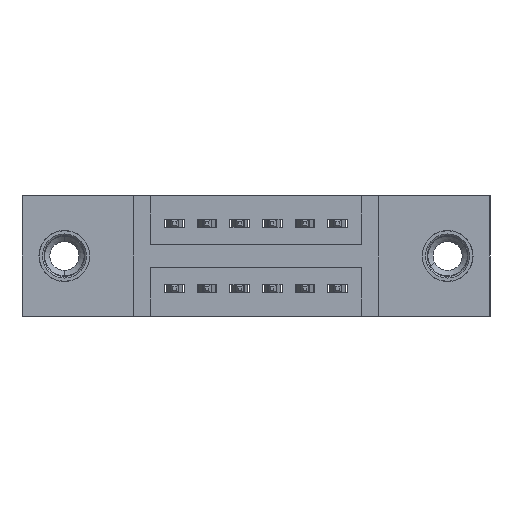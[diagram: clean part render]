
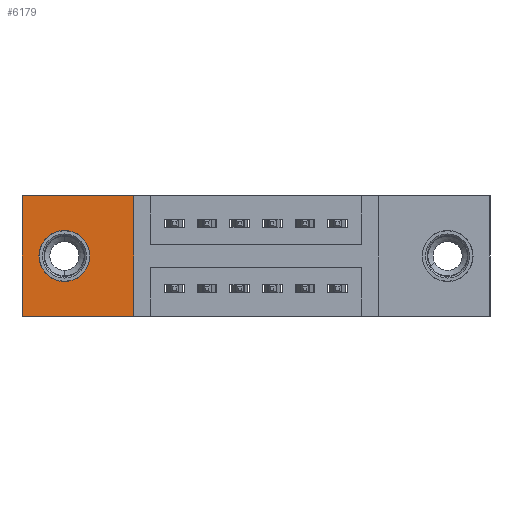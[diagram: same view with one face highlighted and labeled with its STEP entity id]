
A CAD part, front view. The second image highlights one B-rep face of the part: STEP entity #6179.
In plain terms, the highlighted planar face has unit normal (0, -1, 0).
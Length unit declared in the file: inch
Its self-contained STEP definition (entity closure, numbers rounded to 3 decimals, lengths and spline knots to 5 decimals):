
#8 = VERTEX_POINT ( 'NONE', #7902 ) ;
#120 = ORIENTED_EDGE ( 'NONE', *, *, #2230, .T. ) ;
#136 = CARTESIAN_POINT ( 'NONE',  ( 0.13, 0.17, -0.107 ) ) ;
#150 = EDGE_CURVE ( 'NONE', #256, #1971, #10466, .T. ) ;
#256 = VERTEX_POINT ( 'NONE', #9198 ) ;
#309 = EDGE_CURVE ( 'NONE', #10629, #8, #4526, .T. ) ;
#432 = CARTESIAN_POINT ( 'NONE',  ( 0.13, 0.17, -0.185 ) ) ;
#442 = DIRECTION ( 'NONE',  ( 0., 0., -1. ) ) ;
#707 = ORIENTED_EDGE ( 'NONE', *, *, #1881, .T. ) ;
#917 = EDGE_LOOP ( 'NONE', ( #5209, #6041 ) ) ;
#1339 = DIRECTION ( 'NONE',  ( 0., 0., -1. ) ) ;
#1350 = CIRCLE ( 'NONE', #8942, 0.078 ) ;
#1799 = AXIS2_PLACEMENT_3D ( 'NONE', #432, #6364, #1339 ) ;
#1854 = DIRECTION ( 'NONE',  ( 1., 0., 0. ) ) ;
#1881 = EDGE_CURVE ( 'NONE', #1971, #10629, #9957, .T. ) ;
#1959 = CARTESIAN_POINT ( 'NONE',  ( 0., 0.17, 0. ) ) ;
#1971 = VERTEX_POINT ( 'NONE', #9524 ) ;
#2230 = EDGE_CURVE ( 'NONE', #8, #256, #10437, .T. ) ;
#2264 = VECTOR ( 'NONE', #2367, 39.37008 ) ;
#2367 = DIRECTION ( 'NONE',  ( -1., 0., 0. ) ) ;
#2865 = FACE_BOUND ( 'NONE', #917, .T. ) ;
#3296 = VECTOR ( 'NONE', #10123, 39.37008 ) ;
#3959 = EDGE_LOOP ( 'NONE', ( #120, #6352, #707, #6224 ) ) ;
#4275 = EDGE_CURVE ( 'NONE', #10114, #7738, #10608, .T. ) ;
#4370 = DIRECTION ( 'NONE',  ( 0., -1., 0. ) ) ;
#4526 = LINE ( 'NONE', #1959, #2264 ) ;
#4728 = CARTESIAN_POINT ( 'NONE',  ( 0., 0.17, -0.37 ) ) ;
#5209 = ORIENTED_EDGE ( 'NONE', *, *, #4275, .F. ) ;
#5547 = DIRECTION ( 'NONE',  ( 0., -1., 0. ) ) ;
#5842 = CARTESIAN_POINT ( 'NONE',  ( 0.13, 0.17, -0.263 ) ) ;
#6029 = VECTOR ( 'NONE', #8184, 39.37008 ) ;
#6041 = ORIENTED_EDGE ( 'NONE', *, *, #10019, .F. ) ;
#6045 = CARTESIAN_POINT ( 'NONE',  ( 0., 0.17, -0.37 ) ) ;
#6057 = VECTOR ( 'NONE', #1854, 39.37008 ) ;
#6179 = ADVANCED_FACE ( 'NONE', ( #2865, #7611 ), #9695, .T. ) ;
#6224 = ORIENTED_EDGE ( 'NONE', *, *, #309, .T. ) ;
#6352 = ORIENTED_EDGE ( 'NONE', *, *, #150, .T. ) ;
#6364 = DIRECTION ( 'NONE',  ( 0., -1., 0. ) ) ;
#7611 = FACE_OUTER_BOUND ( 'NONE', #3959, .T. ) ;
#7738 = VERTEX_POINT ( 'NONE', #5842 ) ;
#7902 = CARTESIAN_POINT ( 'NONE',  ( 0., 0.17, 0. ) ) ;
#8115 = CARTESIAN_POINT ( 'NONE',  ( 0., 0.17, 0. ) ) ;
#8184 = DIRECTION ( 'NONE',  ( 0., 0., -1. ) ) ;
#8942 = AXIS2_PLACEMENT_3D ( 'NONE', #9331, #4370, #10169 ) ;
#9198 = CARTESIAN_POINT ( 'NONE',  ( 0., 0.17, -0.37 ) ) ;
#9331 = CARTESIAN_POINT ( 'NONE',  ( 0.13, 0.17, -0.185 ) ) ;
#9524 = CARTESIAN_POINT ( 'NONE',  ( 0.3425, 0.17, -0.37 ) ) ;
#9695 = PLANE ( 'NONE',  #10568 ) ;
#9945 = CARTESIAN_POINT ( 'NONE',  ( 0.3425, 0.17, 0. ) ) ;
#9957 = LINE ( 'NONE', #9945, #3296 ) ;
#10019 = EDGE_CURVE ( 'NONE', #7738, #10114, #1350, .T. ) ;
#10114 = VERTEX_POINT ( 'NONE', #136 ) ;
#10123 = DIRECTION ( 'NONE',  ( 0., 0., 1. ) ) ;
#10159 = CARTESIAN_POINT ( 'NONE',  ( 0.3425, 0.17, 0. ) ) ;
#10169 = DIRECTION ( 'NONE',  ( 0., 0., -1. ) ) ;
#10437 = LINE ( 'NONE', #8115, #6029 ) ;
#10466 = LINE ( 'NONE', #6045, #6057 ) ;
#10568 = AXIS2_PLACEMENT_3D ( 'NONE', #4728, #5547, #442 ) ;
#10608 = CIRCLE ( 'NONE', #1799, 0.078 ) ;
#10629 = VERTEX_POINT ( 'NONE', #10159 ) ;
